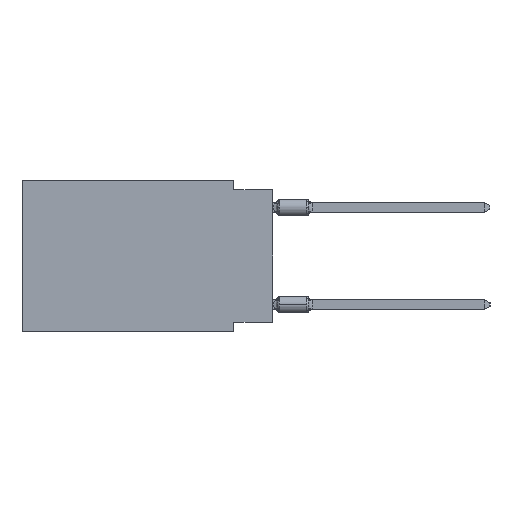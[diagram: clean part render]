
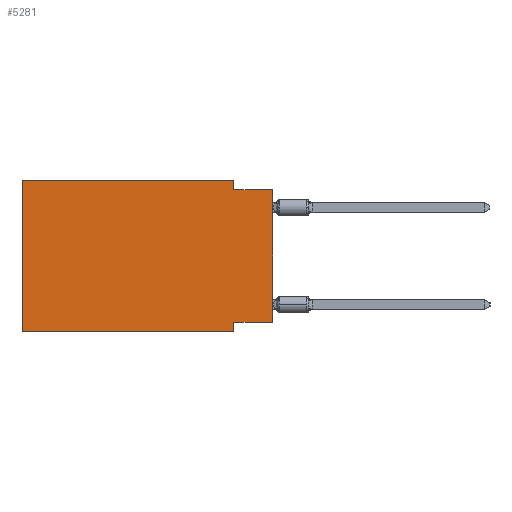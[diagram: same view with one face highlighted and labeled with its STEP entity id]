
A CAD part, left-side view. The second image highlights one B-rep face of the part: STEP entity #5281.
In plain terms, the highlighted planar face has unit normal (-1, 0, 0).
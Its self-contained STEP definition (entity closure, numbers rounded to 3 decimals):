
#2033 = VERTEX_POINT ( 'NONE', #16037 ) ;
#2323 = ORIENTED_EDGE ( 'NONE', *, *, #30418, .T. ) ;
#2443 = ORIENTED_EDGE ( 'NONE', *, *, #17338, .F. ) ;
#2881 = VERTEX_POINT ( 'NONE', #17604 ) ;
#3527 = CARTESIAN_POINT ( 'NONE',  ( 0., 16.383, 0. ) ) ;
#3607 = ORIENTED_EDGE ( 'NONE', *, *, #31155, .F. ) ;
#3975 = VERTEX_POINT ( 'NONE', #21573 ) ;
#5005 = LINE ( 'NONE', #18943, #40461 ) ;
#5281 = ADVANCED_FACE ( 'NONE', ( #9584 ), #26199, .F. ) ;
#6664 = VERTEX_POINT ( 'NONE', #30401 ) ;
#7105 = VECTOR ( 'NONE', #8737, 1000. ) ;
#8737 = DIRECTION ( 'NONE',  ( 0., -1., 0. ) ) ;
#9584 = FACE_OUTER_BOUND ( 'NONE', #22923, .T. ) ;
#10397 = VECTOR ( 'NONE', #18723, 1000. ) ;
#10755 = LINE ( 'NONE', #14088, #17304 ) ;
#12046 = LINE ( 'NONE', #25566, #7105 ) ;
#12056 = CARTESIAN_POINT ( 'NONE',  ( 0., 16.383, 0. ) ) ;
#12310 = ORIENTED_EDGE ( 'NONE', *, *, #18423, .F. ) ;
#13051 = DIRECTION ( 'NONE',  ( 0., -1., 0. ) ) ;
#13708 = LINE ( 'NONE', #3527, #25688 ) ;
#14088 = CARTESIAN_POINT ( 'NONE',  ( 0., 0., -0.635 ) ) ;
#14671 = VERTEX_POINT ( 'NONE', #30830 ) ;
#15075 = ORIENTED_EDGE ( 'NONE', *, *, #32585, .F. ) ;
#15191 = LINE ( 'NONE', #12056, #10397 ) ;
#16037 = CARTESIAN_POINT ( 'NONE',  ( 0., 2.54, -0.635 ) ) ;
#17304 = VECTOR ( 'NONE', #27601, 1000. ) ;
#17338 = EDGE_CURVE ( 'NONE', #31376, #26528, #15191, .T. ) ;
#17604 = CARTESIAN_POINT ( 'NONE',  ( 0., 2.54, 0. ) ) ;
#17667 = CARTESIAN_POINT ( 'NONE',  ( 0., 0., -9.271 ) ) ;
#18423 = EDGE_CURVE ( 'NONE', #26528, #2881, #13708, .T. ) ;
#18723 = DIRECTION ( 'NONE',  ( 0., 0., 1. ) ) ;
#18943 = CARTESIAN_POINT ( 'NONE',  ( 0., 2.54, -9.906 ) ) ;
#19598 = CARTESIAN_POINT ( 'NONE',  ( 0., 16.383, 0. ) ) ;
#19658 = CARTESIAN_POINT ( 'NONE',  ( 0., 0., 0. ) ) ;
#20036 = ORIENTED_EDGE ( 'NONE', *, *, #32232, .T. ) ;
#21573 = CARTESIAN_POINT ( 'NONE',  ( 0., 0., -0.635 ) ) ;
#21883 = LINE ( 'NONE', #19658, #37614 ) ;
#22377 = ORIENTED_EDGE ( 'NONE', *, *, #43623, .F. ) ;
#22923 = EDGE_LOOP ( 'NONE', ( #20036, #31574, #22377, #12310, #2443, #2323, #15075, #3607 ) ) ;
#24008 = DIRECTION ( 'NONE',  ( 0., 0., -1. ) ) ;
#24497 = DIRECTION ( 'NONE',  ( 0., 1., 0. ) ) ;
#25566 = CARTESIAN_POINT ( 'NONE',  ( 0., 16.383, -9.906 ) ) ;
#25688 = VECTOR ( 'NONE', #13051, 1000. ) ;
#26199 = PLANE ( 'NONE',  #42300 ) ;
#26260 = VECTOR ( 'NONE', #24008, 1000. ) ;
#26296 = DIRECTION ( 'NONE',  ( 0., 0., 1. ) ) ;
#26528 = VERTEX_POINT ( 'NONE', #19598 ) ;
#26797 = VERTEX_POINT ( 'NONE', #17667 ) ;
#26937 = CARTESIAN_POINT ( 'NONE',  ( 0., 0., -9.271 ) ) ;
#27601 = DIRECTION ( 'NONE',  ( 0., -1., 0. ) ) ;
#28693 = CARTESIAN_POINT ( 'NONE',  ( 0., 16.383, -9.906 ) ) ;
#28878 = DIRECTION ( 'NONE',  ( 1., 0., 0. ) ) ;
#30401 = CARTESIAN_POINT ( 'NONE',  ( 0., 2.54, -9.271 ) ) ;
#30418 = EDGE_CURVE ( 'NONE', #31376, #14671, #12046, .T. ) ;
#30830 = CARTESIAN_POINT ( 'NONE',  ( 0., 2.54, -9.906 ) ) ;
#31155 = EDGE_CURVE ( 'NONE', #26797, #6664, #43782, .T. ) ;
#31376 = VERTEX_POINT ( 'NONE', #28693 ) ;
#31574 = ORIENTED_EDGE ( 'NONE', *, *, #36531, .F. ) ;
#32232 = EDGE_CURVE ( 'NONE', #26797, #3975, #21883, .T. ) ;
#32585 = EDGE_CURVE ( 'NONE', #6664, #14671, #5005, .T. ) ;
#32593 = VECTOR ( 'NONE', #24497, 1000. ) ;
#32847 = CARTESIAN_POINT ( 'NONE',  ( 0., 16.383, 0. ) ) ;
#34201 = LINE ( 'NONE', #37530, #26260 ) ;
#36531 = EDGE_CURVE ( 'NONE', #2033, #3975, #10755, .T. ) ;
#37530 = CARTESIAN_POINT ( 'NONE',  ( 0., 2.54, 0. ) ) ;
#37614 = VECTOR ( 'NONE', #26296, 1000. ) ;
#40461 = VECTOR ( 'NONE', #41573, 1000. ) ;
#41573 = DIRECTION ( 'NONE',  ( 0., 0., -1. ) ) ;
#42300 = AXIS2_PLACEMENT_3D ( 'NONE', #32847, #28878, #42601 ) ;
#42601 = DIRECTION ( 'NONE',  ( 0., 0., -1. ) ) ;
#43623 = EDGE_CURVE ( 'NONE', #2881, #2033, #34201, .T. ) ;
#43782 = LINE ( 'NONE', #26937, #32593 ) ;
